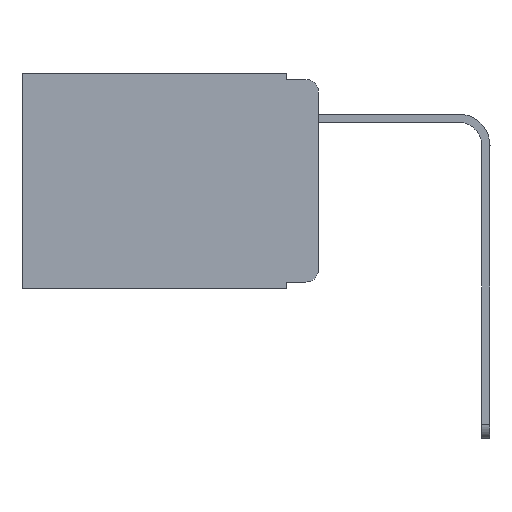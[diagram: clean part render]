
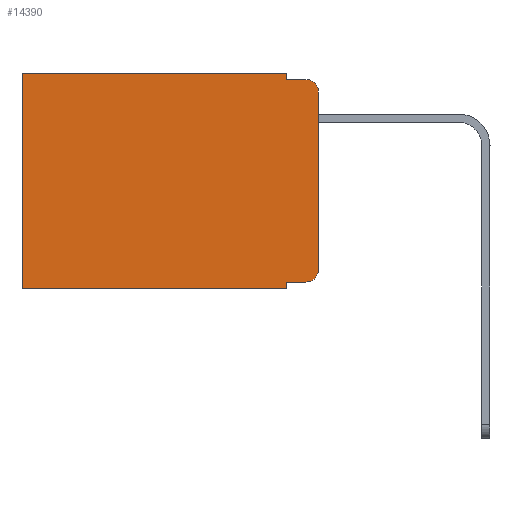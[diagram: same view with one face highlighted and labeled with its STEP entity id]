
A CAD part, left-side view. The second image highlights one B-rep face of the part: STEP entity #14390.
In plain terms, the highlighted planar face has unit normal (-1, 0, 0).
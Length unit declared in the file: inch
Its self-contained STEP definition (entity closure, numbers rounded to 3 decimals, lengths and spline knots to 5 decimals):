
#354 = CARTESIAN_POINT ( 'NONE',  ( 0.298, 0.473, -0.343 ) ) ;
#807 = DIRECTION ( 'NONE',  ( 1., 0., 0. ) ) ;
#993 = DIRECTION ( 'NONE',  ( 0., 0., -1. ) ) ;
#1283 = LINE ( 'NONE', #7033, #4841 ) ;
#1390 = CARTESIAN_POINT ( 'NONE',  ( 0.298, 0., 0. ) ) ;
#1548 = VERTEX_POINT ( 'NONE', #15861 ) ;
#1943 = EDGE_CURVE ( 'NONE', #1548, #16969, #11755, .T. ) ;
#2126 = VERTEX_POINT ( 'NONE', #6436 ) ;
#2142 = EDGE_CURVE ( 'NONE', #13059, #15439, #9358, .T. ) ;
#2213 = CARTESIAN_POINT ( 'NONE',  ( 0.298, 0., 0. ) ) ;
#2398 = EDGE_CURVE ( 'NONE', #2126, #16044, #11255, .T. ) ;
#2404 = VECTOR ( 'NONE', #15006, 39.37008 ) ;
#4318 = VERTEX_POINT ( 'NONE', #9108 ) ;
#4621 = AXIS2_PLACEMENT_3D ( 'NONE', #9416, #15448, #6548 ) ;
#4841 = VECTOR ( 'NONE', #6846, 39.37008 ) ;
#5013 = DIRECTION ( 'NONE',  ( 0., -1., 0. ) ) ;
#5251 = ORIENTED_EDGE ( 'NONE', *, *, #2142, .T. ) ;
#5470 = DIRECTION ( 'NONE',  ( -1., 0., 0. ) ) ;
#5642 = ORIENTED_EDGE ( 'NONE', *, *, #8553, .F. ) ;
#5792 = LINE ( 'NONE', #10291, #19363 ) ;
#6169 = ORIENTED_EDGE ( 'NONE', *, *, #2398, .T. ) ;
#6436 = CARTESIAN_POINT ( 'NONE',  ( 0.298, 0., -0.03 ) ) ;
#6548 = DIRECTION ( 'NONE',  ( 0., 0., -1. ) ) ;
#6741 = PLANE ( 'NONE',  #15279 ) ;
#6846 = DIRECTION ( 'NONE',  ( 0., -1., 0. ) ) ;
#6960 = LINE ( 'NONE', #10930, #9573 ) ;
#7015 = DIRECTION ( 'NONE',  ( 0., 0., -1. ) ) ;
#7033 = CARTESIAN_POINT ( 'NONE',  ( 0.298, 0.051, -0.01 ) ) ;
#7071 = CARTESIAN_POINT ( 'NONE',  ( 0.298, 0.051, -0.333 ) ) ;
#7241 = CARTESIAN_POINT ( 'NONE',  ( 0.298, 0.051, -0.01 ) ) ;
#7545 = EDGE_CURVE ( 'NONE', #16969, #16044, #1283, .T. ) ;
#7613 = ORIENTED_EDGE ( 'NONE', *, *, #8964, .F. ) ;
#7943 = VERTEX_POINT ( 'NONE', #9491 ) ;
#8103 = EDGE_CURVE ( 'NONE', #17367, #11091, #13164, .T. ) ;
#8127 = CARTESIAN_POINT ( 'NONE',  ( 0.298, 0., 0. ) ) ;
#8469 = DIRECTION ( 'NONE',  ( 0., 0., -1. ) ) ;
#8542 = CIRCLE ( 'NONE', #4621, 0.02 ) ;
#8553 = EDGE_CURVE ( 'NONE', #7943, #11091, #6960, .T. ) ;
#8964 = EDGE_CURVE ( 'NONE', #2126, #4318, #15068, .T. ) ;
#9038 = LINE ( 'NONE', #8127, #16202 ) ;
#9054 = EDGE_LOOP ( 'NONE', ( #7613, #6169, #11720, #12580, #18047, #10427, #5642, #13410, #5251, #12900 ) ) ;
#9108 = CARTESIAN_POINT ( 'NONE',  ( 0.298, 0., -0.313 ) ) ;
#9358 = LINE ( 'NONE', #11015, #16061 ) ;
#9416 = CARTESIAN_POINT ( 'NONE',  ( 0.298, 0.02, -0.313 ) ) ;
#9491 = CARTESIAN_POINT ( 'NONE',  ( 0.298, 0.051, -0.343 ) ) ;
#9551 = DIRECTION ( 'NONE',  ( 0., 0., -1. ) ) ;
#9573 = VECTOR ( 'NONE', #18697, 39.37008 ) ;
#9593 = VECTOR ( 'NONE', #9551, 39.37008 ) ;
#9644 = DIRECTION ( 'NONE',  ( 0., 1., 0. ) ) ;
#10291 = CARTESIAN_POINT ( 'NONE',  ( 0.298, 0.051, 0. ) ) ;
#10427 = ORIENTED_EDGE ( 'NONE', *, *, #8103, .T. ) ;
#10930 = CARTESIAN_POINT ( 'NONE',  ( 0.298, 0., -0.343 ) ) ;
#11015 = CARTESIAN_POINT ( 'NONE',  ( 0.298, 0.051, -0.333 ) ) ;
#11091 = VERTEX_POINT ( 'NONE', #354 ) ;
#11137 = CARTESIAN_POINT ( 'NONE',  ( 0.298, 0.02, -0.01 ) ) ;
#11255 = CIRCLE ( 'NONE', #17002, 0.02 ) ;
#11720 = ORIENTED_EDGE ( 'NONE', *, *, #7545, .F. ) ;
#11755 = LINE ( 'NONE', #19151, #12482 ) ;
#11882 = EDGE_CURVE ( 'NONE', #1548, #17367, #9038, .T. ) ;
#12482 = VECTOR ( 'NONE', #993, 39.37008 ) ;
#12580 = ORIENTED_EDGE ( 'NONE', *, *, #1943, .F. ) ;
#12815 = EDGE_CURVE ( 'NONE', #15439, #4318, #8542, .T. ) ;
#12816 = CARTESIAN_POINT ( 'NONE',  ( 0.298, 0.473, 0. ) ) ;
#12900 = ORIENTED_EDGE ( 'NONE', *, *, #12815, .T. ) ;
#13059 = VERTEX_POINT ( 'NONE', #7071 ) ;
#13164 = LINE ( 'NONE', #12816, #9593 ) ;
#13410 = ORIENTED_EDGE ( 'NONE', *, *, #15230, .F. ) ;
#14390 = ADVANCED_FACE ( 'NONE', ( #19389 ), #6741, .F. ) ;
#15006 = DIRECTION ( 'NONE',  ( 0., 0., -1. ) ) ;
#15068 = LINE ( 'NONE', #1390, #2404 ) ;
#15230 = EDGE_CURVE ( 'NONE', #13059, #7943, #5792, .T. ) ;
#15279 = AXIS2_PLACEMENT_3D ( 'NONE', #2213, #807, #8469 ) ;
#15439 = VERTEX_POINT ( 'NONE', #16934 ) ;
#15448 = DIRECTION ( 'NONE',  ( -1., 0., 0. ) ) ;
#15861 = CARTESIAN_POINT ( 'NONE',  ( 0.298, 0.051, 0. ) ) ;
#16044 = VERTEX_POINT ( 'NONE', #11137 ) ;
#16061 = VECTOR ( 'NONE', #5013, 39.37008 ) ;
#16202 = VECTOR ( 'NONE', #9644, 39.37008 ) ;
#16934 = CARTESIAN_POINT ( 'NONE',  ( 0.298, 0.02, -0.333 ) ) ;
#16969 = VERTEX_POINT ( 'NONE', #7241 ) ;
#17002 = AXIS2_PLACEMENT_3D ( 'NONE', #17817, #5470, #7015 ) ;
#17367 = VERTEX_POINT ( 'NONE', #19484 ) ;
#17817 = CARTESIAN_POINT ( 'NONE',  ( 0.298, 0.02, -0.03 ) ) ;
#18016 = DIRECTION ( 'NONE',  ( 0., 0., -1. ) ) ;
#18047 = ORIENTED_EDGE ( 'NONE', *, *, #11882, .T. ) ;
#18697 = DIRECTION ( 'NONE',  ( 0., 1., 0. ) ) ;
#19151 = CARTESIAN_POINT ( 'NONE',  ( 0.298, 0.051, 0. ) ) ;
#19363 = VECTOR ( 'NONE', #18016, 39.37008 ) ;
#19389 = FACE_OUTER_BOUND ( 'NONE', #9054, .T. ) ;
#19484 = CARTESIAN_POINT ( 'NONE',  ( 0.298, 0.473, 0. ) ) ;
